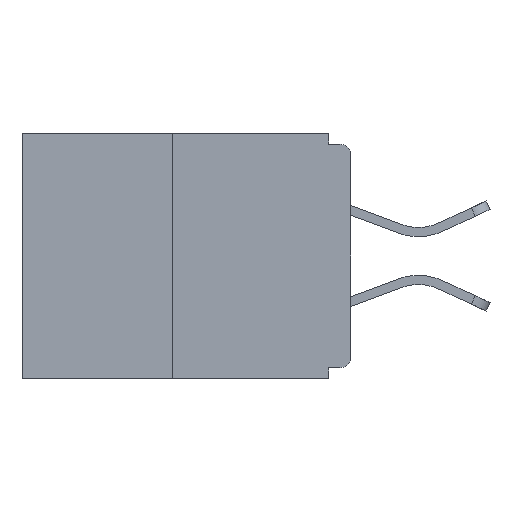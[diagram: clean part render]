
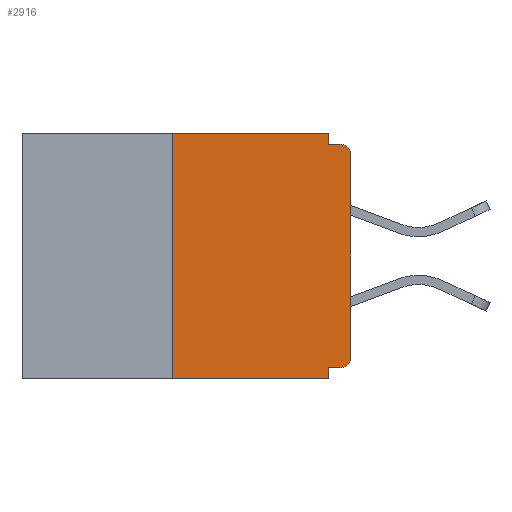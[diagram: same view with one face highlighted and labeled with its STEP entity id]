
A CAD part, left-side view. The second image highlights one B-rep face of the part: STEP entity #2916.
In plain terms, the highlighted planar face has unit normal (-1, 0, 0).
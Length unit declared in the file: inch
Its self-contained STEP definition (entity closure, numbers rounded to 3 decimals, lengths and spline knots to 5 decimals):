
#202 = CARTESIAN_POINT ( 'NONE',  ( 0., 0., -0.015 ) ) ;
#688 = VECTOR ( 'NONE', #5299, 39.37008 ) ;
#1038 = DIRECTION ( 'NONE',  ( 0., 0., -1. ) ) ;
#1135 = ORIENTED_EDGE ( 'NONE', *, *, #9589, .F. ) ;
#1137 = CARTESIAN_POINT ( 'NONE',  ( 0., 0.25, 0. ) ) ;
#1438 = DIRECTION ( 'NONE',  ( 0., -1., 0. ) ) ;
#1481 = EDGE_CURVE ( 'NONE', #1800, #14599, #11040, .T. ) ;
#1772 = VECTOR ( 'NONE', #10933, 39.37008 ) ;
#1800 = VERTEX_POINT ( 'NONE', #2923 ) ;
#2154 = VERTEX_POINT ( 'NONE', #10932 ) ;
#2458 = VERTEX_POINT ( 'NONE', #14012 ) ;
#2803 = AXIS2_PLACEMENT_3D ( 'NONE', #9776, #15913, #1038 ) ;
#2916 = ADVANCED_FACE ( 'NONE', ( #14068 ), #5846, .F. ) ;
#2923 = CARTESIAN_POINT ( 'NONE',  ( 0., 0.25, -0.343 ) ) ;
#3403 = DIRECTION ( 'NONE',  ( 1., 0., 0. ) ) ;
#3658 = EDGE_CURVE ( 'NONE', #7520, #11648, #14434, .T. ) ;
#4077 = VERTEX_POINT ( 'NONE', #6514 ) ;
#4495 = VECTOR ( 'NONE', #5915, 39.37008 ) ;
#4622 = CARTESIAN_POINT ( 'NONE',  ( 0., 0.015, -0.328 ) ) ;
#4967 = CARTESIAN_POINT ( 'NONE',  ( 0., 0., -0.328 ) ) ;
#5027 = VECTOR ( 'NONE', #7412, 39.37008 ) ;
#5028 = CARTESIAN_POINT ( 'NONE',  ( 0., 0., -0.313 ) ) ;
#5088 = CARTESIAN_POINT ( 'NONE',  ( 0., 0., -0.03 ) ) ;
#5133 = ORIENTED_EDGE ( 'NONE', *, *, #6876, .T. ) ;
#5299 = DIRECTION ( 'NONE',  ( 0., 0., -1. ) ) ;
#5482 = CARTESIAN_POINT ( 'NONE',  ( 0., 0.031, 0. ) ) ;
#5687 = LINE ( 'NONE', #5482, #14357 ) ;
#5783 = ORIENTED_EDGE ( 'NONE', *, *, #12645, .F. ) ;
#5846 = PLANE ( 'NONE',  #6731 ) ;
#5915 = DIRECTION ( 'NONE',  ( 0., -1., 0. ) ) ;
#6014 = EDGE_CURVE ( 'NONE', #7715, #6015, #11615, .T. ) ;
#6015 = VERTEX_POINT ( 'NONE', #10078 ) ;
#6251 = LINE ( 'NONE', #12594, #688 ) ;
#6509 = EDGE_CURVE ( 'NONE', #7520, #2458, #7533, .T. ) ;
#6514 = CARTESIAN_POINT ( 'NONE',  ( 0., 0.031, 0. ) ) ;
#6675 = DIRECTION ( 'NONE',  ( 0., 1., 0. ) ) ;
#6731 = AXIS2_PLACEMENT_3D ( 'NONE', #10776, #3403, #15684 ) ;
#6876 = EDGE_CURVE ( 'NONE', #1800, #2154, #11966, .T. ) ;
#7237 = CARTESIAN_POINT ( 'NONE',  ( 0., 0.015, -0.03 ) ) ;
#7412 = DIRECTION ( 'NONE',  ( 0., -1., 0. ) ) ;
#7520 = VERTEX_POINT ( 'NONE', #4622 ) ;
#7533 = LINE ( 'NONE', #4967, #10260 ) ;
#7715 = VERTEX_POINT ( 'NONE', #14533 ) ;
#7780 = LINE ( 'NONE', #15805, #4495 ) ;
#8039 = EDGE_LOOP ( 'NONE', ( #5783, #13331, #5133, #15751, #12860, #13482, #8056, #9642, #13593, #1135 ) ) ;
#8056 = ORIENTED_EDGE ( 'NONE', *, *, #14290, .T. ) ;
#8186 = AXIS2_PLACEMENT_3D ( 'NONE', #7237, #10944, #9873 ) ;
#8715 = VECTOR ( 'NONE', #9777, 39.37008 ) ;
#8729 = LINE ( 'NONE', #11099, #1772 ) ;
#9589 = EDGE_CURVE ( 'NONE', #4077, #7715, #5687, .T. ) ;
#9642 = ORIENTED_EDGE ( 'NONE', *, *, #11273, .T. ) ;
#9776 = CARTESIAN_POINT ( 'NONE',  ( 0., 0.015, -0.313 ) ) ;
#9777 = DIRECTION ( 'NONE',  ( 0., 0., 1. ) ) ;
#9793 = CIRCLE ( 'NONE', #8186, 0.015 ) ;
#9873 = DIRECTION ( 'NONE',  ( 0., 0., -1. ) ) ;
#9999 = EDGE_CURVE ( 'NONE', #2458, #2154, #6251, .T. ) ;
#10078 = CARTESIAN_POINT ( 'NONE',  ( 0., 0.015, -0.015 ) ) ;
#10260 = VECTOR ( 'NONE', #6675, 39.37008 ) ;
#10776 = CARTESIAN_POINT ( 'NONE',  ( 0., 0.46, 0. ) ) ;
#10932 = CARTESIAN_POINT ( 'NONE',  ( 0., 0.031, -0.343 ) ) ;
#10933 = DIRECTION ( 'NONE',  ( 0., 0., 1. ) ) ;
#10944 = DIRECTION ( 'NONE',  ( -1., 0., 0. ) ) ;
#11040 = LINE ( 'NONE', #1137, #8715 ) ;
#11059 = CARTESIAN_POINT ( 'NONE',  ( 0., 0.46, -0.343 ) ) ;
#11099 = CARTESIAN_POINT ( 'NONE',  ( 0., 0., 0. ) ) ;
#11273 = EDGE_CURVE ( 'NONE', #15768, #6015, #9793, .T. ) ;
#11615 = LINE ( 'NONE', #202, #14493 ) ;
#11648 = VERTEX_POINT ( 'NONE', #5028 ) ;
#11966 = LINE ( 'NONE', #11059, #5027 ) ;
#12594 = CARTESIAN_POINT ( 'NONE',  ( 0., 0.031, -0.343 ) ) ;
#12645 = EDGE_CURVE ( 'NONE', #14599, #4077, #7780, .T. ) ;
#12860 = ORIENTED_EDGE ( 'NONE', *, *, #6509, .F. ) ;
#13331 = ORIENTED_EDGE ( 'NONE', *, *, #1481, .F. ) ;
#13482 = ORIENTED_EDGE ( 'NONE', *, *, #3658, .T. ) ;
#13593 = ORIENTED_EDGE ( 'NONE', *, *, #6014, .F. ) ;
#14012 = CARTESIAN_POINT ( 'NONE',  ( 0., 0.031, -0.328 ) ) ;
#14068 = FACE_OUTER_BOUND ( 'NONE', #8039, .T. ) ;
#14149 = DIRECTION ( 'NONE',  ( 0., 0., -1. ) ) ;
#14290 = EDGE_CURVE ( 'NONE', #11648, #15768, #8729, .T. ) ;
#14357 = VECTOR ( 'NONE', #14149, 39.37008 ) ;
#14434 = CIRCLE ( 'NONE', #2803, 0.015 ) ;
#14493 = VECTOR ( 'NONE', #1438, 39.37008 ) ;
#14533 = CARTESIAN_POINT ( 'NONE',  ( 0., 0.031, -0.015 ) ) ;
#14599 = VERTEX_POINT ( 'NONE', #15243 ) ;
#15243 = CARTESIAN_POINT ( 'NONE',  ( 0., 0.25, 0. ) ) ;
#15684 = DIRECTION ( 'NONE',  ( 0., 0., -1. ) ) ;
#15751 = ORIENTED_EDGE ( 'NONE', *, *, #9999, .F. ) ;
#15768 = VERTEX_POINT ( 'NONE', #5088 ) ;
#15805 = CARTESIAN_POINT ( 'NONE',  ( 0., 0.46, 0. ) ) ;
#15913 = DIRECTION ( 'NONE',  ( -1., 0., 0. ) ) ;
